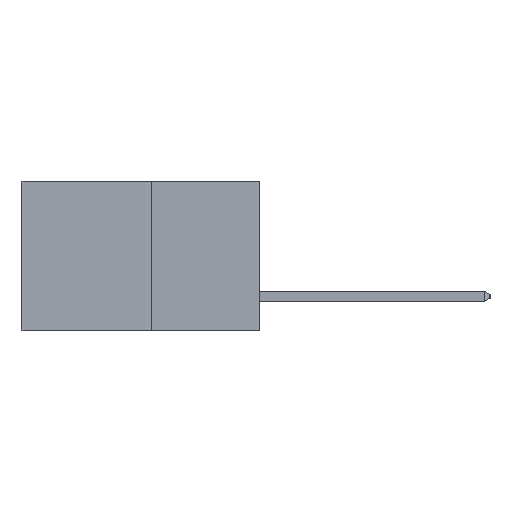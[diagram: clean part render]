
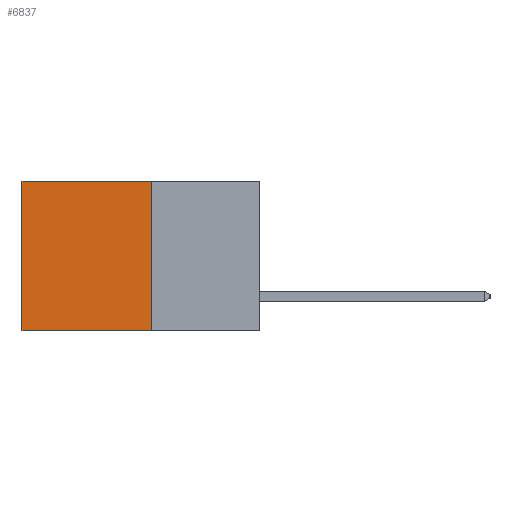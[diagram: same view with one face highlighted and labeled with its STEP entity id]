
A CAD part, left-side view. The second image highlights one B-rep face of the part: STEP entity #6837.
In plain terms, the highlighted planar face has unit normal (-1, 0, 0).
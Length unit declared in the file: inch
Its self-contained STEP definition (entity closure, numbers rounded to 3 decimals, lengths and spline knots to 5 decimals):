
#520 = LINE ( 'NONE', #2277, #2294 ) ;
#727 = ORIENTED_EDGE ( 'NONE', *, *, #2867, .F. ) ;
#762 = CARTESIAN_POINT ( 'NONE',  ( 0.277, 0.27, -0.37 ) ) ;
#1180 = VERTEX_POINT ( 'NONE', #4437 ) ;
#1286 = EDGE_LOOP ( 'NONE', ( #3362, #5577, #727, #1502 ) ) ;
#1502 = ORIENTED_EDGE ( 'NONE', *, *, #3244, .T. ) ;
#1603 = VECTOR ( 'NONE', #5791, 39.37008 ) ;
#1796 = CARTESIAN_POINT ( 'NONE',  ( 0.277, 0.27, -0.37 ) ) ;
#2277 = CARTESIAN_POINT ( 'NONE',  ( 0.277, 0.27, 0. ) ) ;
#2294 = VECTOR ( 'NONE', #3611, 39.37008 ) ;
#2549 = DIRECTION ( 'NONE',  ( 1., 0., 0. ) ) ;
#2867 = EDGE_CURVE ( 'NONE', #3447, #6629, #9269, .T. ) ;
#2918 = DIRECTION ( 'NONE',  ( 0., 1., 0. ) ) ;
#3001 = CARTESIAN_POINT ( 'NONE',  ( 0.277, 0.27, -0.37 ) ) ;
#3235 = CARTESIAN_POINT ( 'NONE',  ( 0.277, 0.59, -0.37 ) ) ;
#3244 = EDGE_CURVE ( 'NONE', #3447, #1180, #520, .T. ) ;
#3296 = EDGE_CURVE ( 'NONE', #6629, #6804, #7585, .T. ) ;
#3362 = ORIENTED_EDGE ( 'NONE', *, *, #8902, .T. ) ;
#3447 = VERTEX_POINT ( 'NONE', #4894 ) ;
#3522 = CARTESIAN_POINT ( 'NONE',  ( 0.277, 0.59, -0.37 ) ) ;
#3611 = DIRECTION ( 'NONE',  ( 0., 1., 0. ) ) ;
#3793 = VECTOR ( 'NONE', #2918, 39.37008 ) ;
#4437 = CARTESIAN_POINT ( 'NONE',  ( 0.277, 0.59, 0. ) ) ;
#4516 = CARTESIAN_POINT ( 'NONE',  ( 0.277, 0.27, -0.37 ) ) ;
#4894 = CARTESIAN_POINT ( 'NONE',  ( 0.277, 0.27, 0. ) ) ;
#4974 = DIRECTION ( 'NONE',  ( 0., 0., -1. ) ) ;
#5504 = VECTOR ( 'NONE', #4974, 39.37008 ) ;
#5577 = ORIENTED_EDGE ( 'NONE', *, *, #3296, .F. ) ;
#5791 = DIRECTION ( 'NONE',  ( 0., 0., -1. ) ) ;
#6150 = AXIS2_PLACEMENT_3D ( 'NONE', #1796, #2549, #7571 ) ;
#6154 = PLANE ( 'NONE',  #6150 ) ;
#6629 = VERTEX_POINT ( 'NONE', #762 ) ;
#6804 = VERTEX_POINT ( 'NONE', #3235 ) ;
#6837 = ADVANCED_FACE ( 'NONE', ( #6857 ), #6154, .F. ) ;
#6857 = FACE_OUTER_BOUND ( 'NONE', #1286, .T. ) ;
#7571 = DIRECTION ( 'NONE',  ( 0., 0., -1. ) ) ;
#7585 = LINE ( 'NONE', #3001, #3793 ) ;
#8902 = EDGE_CURVE ( 'NONE', #1180, #6804, #9275, .T. ) ;
#9269 = LINE ( 'NONE', #4516, #1603 ) ;
#9275 = LINE ( 'NONE', #3522, #5504 ) ;
